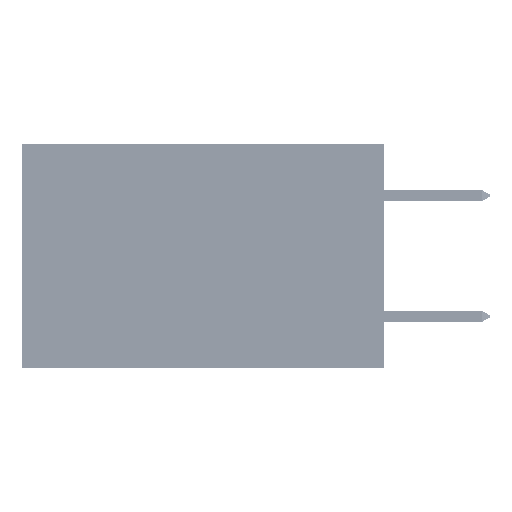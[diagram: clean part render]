
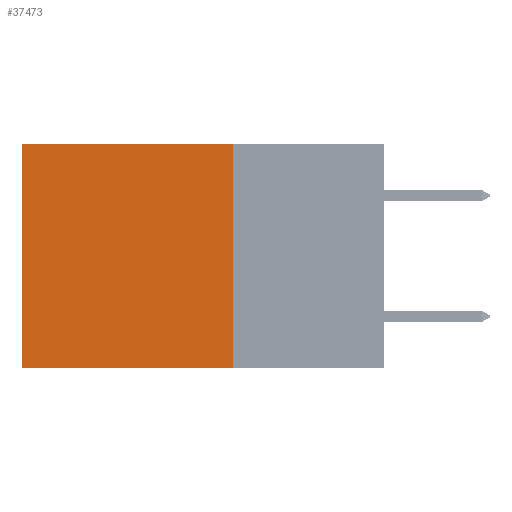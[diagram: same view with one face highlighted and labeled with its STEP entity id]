
A CAD part, left-side view. The second image highlights one B-rep face of the part: STEP entity #37473.
In plain terms, the highlighted planar face has unit normal (-1, 0, 0).
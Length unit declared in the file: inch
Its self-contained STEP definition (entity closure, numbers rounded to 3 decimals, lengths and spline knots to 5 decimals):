
#273 = ORIENTED_EDGE ( 'NONE', *, *, #39573, .F. ) ;
#2934 = DIRECTION ( 'NONE',  ( 0., 0., -1. ) ) ;
#3154 = DIRECTION ( 'NONE',  ( 0., 1., 0. ) ) ;
#4240 = LINE ( 'NONE', #13954, #26989 ) ;
#8527 = DIRECTION ( 'NONE',  ( 0., 0., -1. ) ) ;
#10670 = VECTOR ( 'NONE', #2934, 39.37008 ) ;
#12079 = VECTOR ( 'NONE', #3154, 39.37008 ) ;
#12171 = AXIS2_PLACEMENT_3D ( 'NONE', #26190, #36683, #8527 ) ;
#13716 = CARTESIAN_POINT ( 'NONE',  ( 0.2875, 0.25, 0. ) ) ;
#13954 = CARTESIAN_POINT ( 'NONE',  ( 0.2875, 0.25, 0. ) ) ;
#15320 = VERTEX_POINT ( 'NONE', #13716 ) ;
#15616 = PLANE ( 'NONE',  #12171 ) ;
#16398 = EDGE_CURVE ( 'NONE', #37116, #38992, #44661, .T. ) ;
#17677 = DIRECTION ( 'NONE',  ( 0., 1., 0. ) ) ;
#19831 = FACE_OUTER_BOUND ( 'NONE', #24375, .T. ) ;
#20761 = CARTESIAN_POINT ( 'NONE',  ( 0.2875, 0.6, 0. ) ) ;
#21002 = ORIENTED_EDGE ( 'NONE', *, *, #28045, .T. ) ;
#21526 = LINE ( 'NONE', #32048, #12079 ) ;
#24375 = EDGE_LOOP ( 'NONE', ( #25597, #42473, #273, #21002 ) ) ;
#25169 = VECTOR ( 'NONE', #26359, 39.37008 ) ;
#25597 = ORIENTED_EDGE ( 'NONE', *, *, #16398, .T. ) ;
#26190 = CARTESIAN_POINT ( 'NONE',  ( 0.2875, 0.25, 0. ) ) ;
#26359 = DIRECTION ( 'NONE',  ( 0., 0., -1. ) ) ;
#26989 = VECTOR ( 'NONE', #17677, 39.37008 ) ;
#27443 = EDGE_CURVE ( 'NONE', #31747, #38992, #21526, .T. ) ;
#27938 = LINE ( 'NONE', #33990, #25169 ) ;
#28045 = EDGE_CURVE ( 'NONE', #15320, #37116, #4240, .T. ) ;
#31747 = VERTEX_POINT ( 'NONE', #42896 ) ;
#32048 = CARTESIAN_POINT ( 'NONE',  ( 0.2875, 0.25, -0.37 ) ) ;
#33990 = CARTESIAN_POINT ( 'NONE',  ( 0.2875, 0.25, 0. ) ) ;
#34675 = CARTESIAN_POINT ( 'NONE',  ( 0.2875, 0.6, -0.37 ) ) ;
#36683 = DIRECTION ( 'NONE',  ( 1., 0., 0. ) ) ;
#37116 = VERTEX_POINT ( 'NONE', #39123 ) ;
#37473 = ADVANCED_FACE ( 'NONE', ( #19831 ), #15616, .F. ) ;
#38992 = VERTEX_POINT ( 'NONE', #34675 ) ;
#39123 = CARTESIAN_POINT ( 'NONE',  ( 0.2875, 0.6, 0. ) ) ;
#39573 = EDGE_CURVE ( 'NONE', #15320, #31747, #27938, .T. ) ;
#42473 = ORIENTED_EDGE ( 'NONE', *, *, #27443, .F. ) ;
#42896 = CARTESIAN_POINT ( 'NONE',  ( 0.2875, 0.25, -0.37 ) ) ;
#44661 = LINE ( 'NONE', #20761, #10670 ) ;
